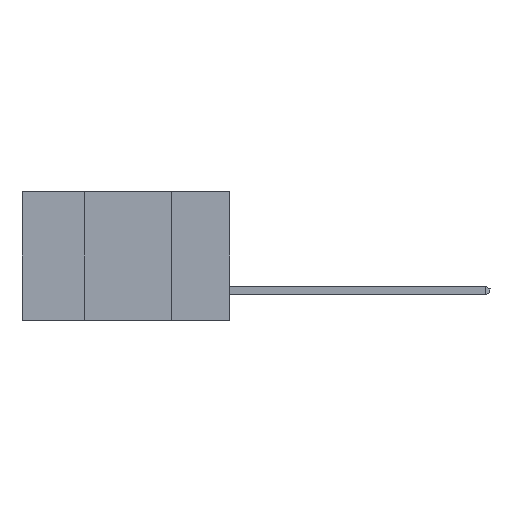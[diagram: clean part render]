
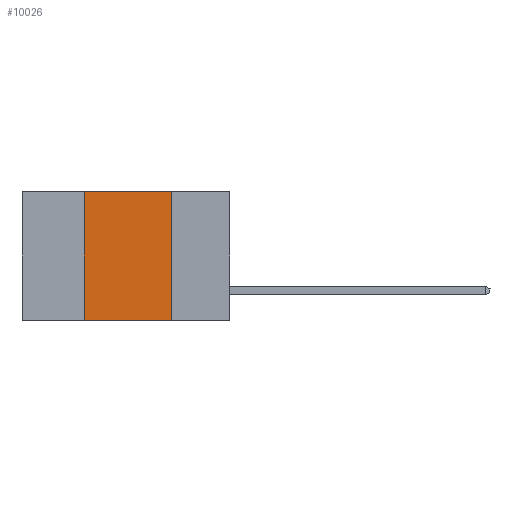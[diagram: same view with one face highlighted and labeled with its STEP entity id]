
A CAD part, left-side view. The second image highlights one B-rep face of the part: STEP entity #10026.
In plain terms, the highlighted planar face has unit normal (-1, 0, 0).
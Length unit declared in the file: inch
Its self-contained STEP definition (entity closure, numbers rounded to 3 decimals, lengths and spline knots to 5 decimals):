
#675 = PLANE ( 'NONE',  #2995 ) ;
#974 = VERTEX_POINT ( 'NONE', #11603 ) ;
#1141 = CARTESIAN_POINT ( 'NONE',  ( 0., 0.17, -0.37 ) ) ;
#1545 = DIRECTION ( 'NONE',  ( 0., 0., 1. ) ) ;
#1921 = ORIENTED_EDGE ( 'NONE', *, *, #13093, .F. ) ;
#2036 = CARTESIAN_POINT ( 'NONE',  ( 0., 0.6, -0.37 ) ) ;
#2670 = VERTEX_POINT ( 'NONE', #12591 ) ;
#2795 = CARTESIAN_POINT ( 'NONE',  ( 0., 0.6, 0. ) ) ;
#2995 = AXIS2_PLACEMENT_3D ( 'NONE', #9991, #15897, #17481 ) ;
#3528 = VERTEX_POINT ( 'NONE', #12081 ) ;
#5536 = VECTOR ( 'NONE', #9422, 39.37008 ) ;
#8521 = DIRECTION ( 'NONE',  ( 0., 0., -1. ) ) ;
#8853 = CARTESIAN_POINT ( 'NONE',  ( 0., 0.17, -0.37 ) ) ;
#9255 = EDGE_CURVE ( 'NONE', #974, #3528, #18500, .T. ) ;
#9422 = DIRECTION ( 'NONE',  ( 0., -1., 0. ) ) ;
#9991 = CARTESIAN_POINT ( 'NONE',  ( 0., 0.6, 0. ) ) ;
#10026 = ADVANCED_FACE ( 'NONE', ( #23054 ), #675, .F. ) ;
#11207 = ORIENTED_EDGE ( 'NONE', *, *, #21422, .F. ) ;
#11603 = CARTESIAN_POINT ( 'NONE',  ( 0., 0.42, -0.37 ) ) ;
#12081 = CARTESIAN_POINT ( 'NONE',  ( 0., 0.42, 0. ) ) ;
#12562 = CARTESIAN_POINT ( 'NONE',  ( 0., 0.42, -0.37 ) ) ;
#12591 = CARTESIAN_POINT ( 'NONE',  ( 0., 0.17, 0. ) ) ;
#13024 = VECTOR ( 'NONE', #8521, 39.37008 ) ;
#13093 = EDGE_CURVE ( 'NONE', #2670, #16993, #17730, .T. ) ;
#13657 = VECTOR ( 'NONE', #19033, 39.37008 ) ;
#15095 = ORIENTED_EDGE ( 'NONE', *, *, #9255, .F. ) ;
#15897 = DIRECTION ( 'NONE',  ( 1., 0., 0. ) ) ;
#16993 = VERTEX_POINT ( 'NONE', #8853 ) ;
#17481 = DIRECTION ( 'NONE',  ( 0., 0., -1. ) ) ;
#17730 = LINE ( 'NONE', #1141, #13024 ) ;
#18500 = LINE ( 'NONE', #12562, #20750 ) ;
#18622 = LINE ( 'NONE', #2036, #5536 ) ;
#19033 = DIRECTION ( 'NONE',  ( 0., -1., 0. ) ) ;
#20599 = EDGE_LOOP ( 'NONE', ( #1921, #11207, #15095, #22434 ) ) ;
#20750 = VECTOR ( 'NONE', #1545, 39.37008 ) ;
#21098 = LINE ( 'NONE', #2795, #13657 ) ;
#21422 = EDGE_CURVE ( 'NONE', #3528, #2670, #21098, .T. ) ;
#22434 = ORIENTED_EDGE ( 'NONE', *, *, #23452, .T. ) ;
#23054 = FACE_OUTER_BOUND ( 'NONE', #20599, .T. ) ;
#23452 = EDGE_CURVE ( 'NONE', #974, #16993, #18622, .T. ) ;
